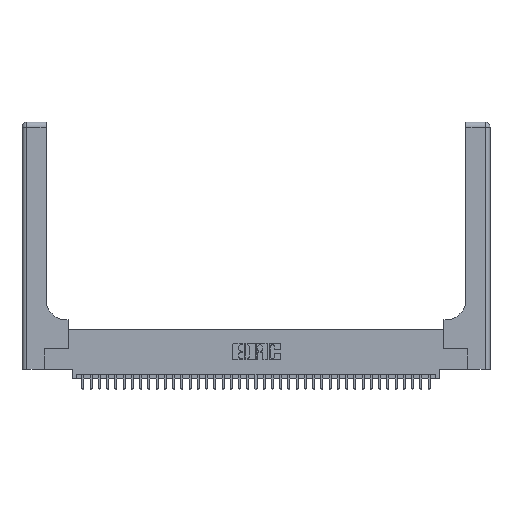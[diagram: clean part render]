
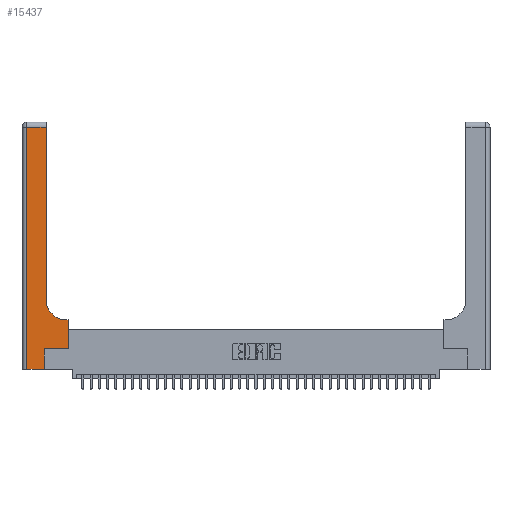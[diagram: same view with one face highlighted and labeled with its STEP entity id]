
A CAD part, top view. The second image highlights one B-rep face of the part: STEP entity #15437.
In plain terms, the highlighted planar face has unit normal (0, 0, 1).
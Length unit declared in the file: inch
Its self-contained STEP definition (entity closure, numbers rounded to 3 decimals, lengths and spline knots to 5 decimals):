
#312 = VECTOR ( 'NONE', #28309, 39.37008 ) ;
#408 = VERTEX_POINT ( 'NONE', #15894 ) ;
#1051 = CARTESIAN_POINT ( 'NONE',  ( 0.269, 0., 0.37 ) ) ;
#1366 = VERTEX_POINT ( 'NONE', #23676 ) ;
#1425 = LINE ( 'NONE', #28928, #16588 ) ;
#2004 = VERTEX_POINT ( 'NONE', #8659 ) ;
#3266 = ORIENTED_EDGE ( 'NONE', *, *, #7566, .T. ) ;
#3683 = EDGE_CURVE ( 'NONE', #12951, #36385, #13857, .T. ) ;
#3761 = ORIENTED_EDGE ( 'NONE', *, *, #33022, .T. ) ;
#4398 = VERTEX_POINT ( 'NONE', #1051 ) ;
#5148 = ORIENTED_EDGE ( 'NONE', *, *, #27526, .T. ) ;
#5382 = DIRECTION ( 'NONE',  ( -1., 0., 0. ) ) ;
#5711 = CARTESIAN_POINT ( 'NONE',  ( 0.269, 0.25, 0.37 ) ) ;
#5830 = VECTOR ( 'NONE', #24543, 39.37008 ) ;
#7566 = EDGE_CURVE ( 'NONE', #13489, #1366, #10328, .T. ) ;
#8070 = CARTESIAN_POINT ( 'NONE',  ( 0.2915, 0.6, 0.37 ) ) ;
#8268 = AXIS2_PLACEMENT_3D ( 'NONE', #27555, #9578, #30545 ) ;
#8633 = CIRCLE ( 'NONE', #8268, 0.25 ) ;
#8643 = VERTEX_POINT ( 'NONE', #15843 ) ;
#8659 = CARTESIAN_POINT ( 'NONE',  ( 0.5585, 0.6, 0.37 ) ) ;
#8951 = ORIENTED_EDGE ( 'NONE', *, *, #22738, .T. ) ;
#9375 = VECTOR ( 'NONE', #28234, 39.37008 ) ;
#9578 = DIRECTION ( 'NONE',  ( 0., 0., -1. ) ) ;
#10328 = LINE ( 'NONE', #34262, #9375 ) ;
#11812 = DIRECTION ( 'NONE',  ( 0., 1., 0. ) ) ;
#12029 = LINE ( 'NONE', #32758, #36877 ) ;
#12640 = CARTESIAN_POINT ( 'NONE',  ( 0., 0., 0.37 ) ) ;
#12951 = VERTEX_POINT ( 'NONE', #5711 ) ;
#13489 = VERTEX_POINT ( 'NONE', #29040 ) ;
#13495 = EDGE_CURVE ( 'NONE', #2004, #8643, #38212, .T. ) ;
#13677 = ORIENTED_EDGE ( 'NONE', *, *, #23597, .T. ) ;
#13857 = LINE ( 'NONE', #30441, #5830 ) ;
#13864 = LINE ( 'NONE', #37220, #312 ) ;
#14123 = DIRECTION ( 'NONE',  ( -1., 0., 0. ) ) ;
#15369 = CARTESIAN_POINT ( 'NONE',  ( 0., 2.94, 0.37 ) ) ;
#15437 = ADVANCED_FACE ( 'NONE', ( #35840 ), #29276, .F. ) ;
#15843 = CARTESIAN_POINT ( 'NONE',  ( 0.5415, 0.6, 0.37 ) ) ;
#15894 = CARTESIAN_POINT ( 'NONE',  ( 0.06, 0., 0.37 ) ) ;
#16588 = VECTOR ( 'NONE', #31962, 39.37008 ) ;
#17497 = VECTOR ( 'NONE', #27563, 39.37008 ) ;
#18058 = EDGE_CURVE ( 'NONE', #1366, #36993, #32329, .T. ) ;
#18847 = ORIENTED_EDGE ( 'NONE', *, *, #3683, .T. ) ;
#20343 = AXIS2_PLACEMENT_3D ( 'NONE', #38345, #23409, #5382 ) ;
#22738 = EDGE_CURVE ( 'NONE', #4398, #12951, #12029, .T. ) ;
#23409 = DIRECTION ( 'NONE',  ( 0., 0., -1. ) ) ;
#23597 = EDGE_CURVE ( 'NONE', #8643, #13489, #8633, .T. ) ;
#23676 = CARTESIAN_POINT ( 'NONE',  ( 0.2915, 2.94, 0.37 ) ) ;
#24383 = VECTOR ( 'NONE', #36318, 39.37008 ) ;
#24512 = LINE ( 'NONE', #12640, #17497 ) ;
#24543 = DIRECTION ( 'NONE',  ( 1., 0., 0. ) ) ;
#27255 = ORIENTED_EDGE ( 'NONE', *, *, #18058, .T. ) ;
#27526 = EDGE_CURVE ( 'NONE', #36993, #408, #13864, .T. ) ;
#27555 = CARTESIAN_POINT ( 'NONE',  ( 0.5415, 0.85, 0.37 ) ) ;
#27563 = DIRECTION ( 'NONE',  ( 1., 0., 0. ) ) ;
#28234 = DIRECTION ( 'NONE',  ( 0., 1., 0. ) ) ;
#28309 = DIRECTION ( 'NONE',  ( 0., -1., 0. ) ) ;
#28355 = VECTOR ( 'NONE', #14123, 39.37008 ) ;
#28779 = CARTESIAN_POINT ( 'NONE',  ( 0.5585, 0.25, 0.37 ) ) ;
#28928 = CARTESIAN_POINT ( 'NONE',  ( 0.5585, 0.25, 0.37 ) ) ;
#29040 = CARTESIAN_POINT ( 'NONE',  ( 0.2915, 0.85, 0.37 ) ) ;
#29100 = ORIENTED_EDGE ( 'NONE', *, *, #35445, .T. ) ;
#29276 = PLANE ( 'NONE',  #20343 ) ;
#30441 = CARTESIAN_POINT ( 'NONE',  ( 0.269, 0.25, 0.37 ) ) ;
#30545 = DIRECTION ( 'NONE',  ( 1., 0., 0. ) ) ;
#31765 = EDGE_LOOP ( 'NONE', ( #3266, #27255, #5148, #29100, #8951, #18847, #3761, #36665, #13677 ) ) ;
#31962 = DIRECTION ( 'NONE',  ( 0., 1., 0. ) ) ;
#32329 = LINE ( 'NONE', #15369, #24383 ) ;
#32758 = CARTESIAN_POINT ( 'NONE',  ( 0.269, 0., 0.37 ) ) ;
#33022 = EDGE_CURVE ( 'NONE', #36385, #2004, #1425, .T. ) ;
#34262 = CARTESIAN_POINT ( 'NONE',  ( 0.2915, 3., 0.37 ) ) ;
#34933 = CARTESIAN_POINT ( 'NONE',  ( 0.06, 2.94, 0.37 ) ) ;
#35445 = EDGE_CURVE ( 'NONE', #408, #4398, #24512, .T. ) ;
#35840 = FACE_OUTER_BOUND ( 'NONE', #31765, .T. ) ;
#36318 = DIRECTION ( 'NONE',  ( -1., 0., 0. ) ) ;
#36385 = VERTEX_POINT ( 'NONE', #28779 ) ;
#36665 = ORIENTED_EDGE ( 'NONE', *, *, #13495, .T. ) ;
#36877 = VECTOR ( 'NONE', #11812, 39.37008 ) ;
#36993 = VERTEX_POINT ( 'NONE', #34933 ) ;
#37220 = CARTESIAN_POINT ( 'NONE',  ( 0.06, 3., 0.37 ) ) ;
#38212 = LINE ( 'NONE', #8070, #28355 ) ;
#38345 = CARTESIAN_POINT ( 'NONE',  ( 0., 3., 0.37 ) ) ;
